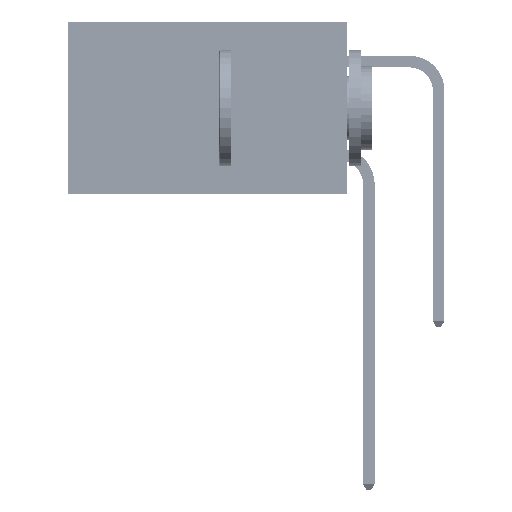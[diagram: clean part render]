
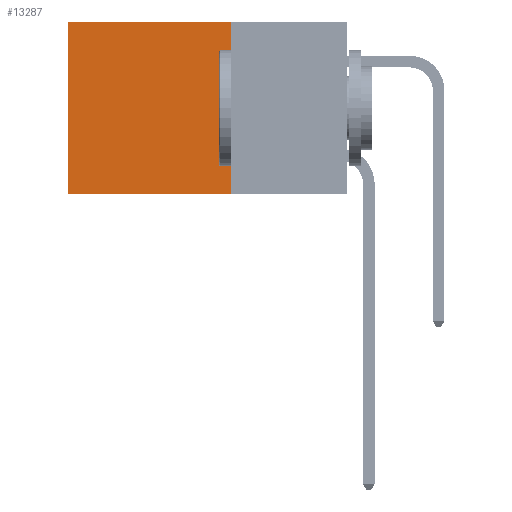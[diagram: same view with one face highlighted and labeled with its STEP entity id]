
A CAD part, left-side view. The second image highlights one B-rep face of the part: STEP entity #13287.
In plain terms, the highlighted planar face has unit normal (-1, 0, 0).
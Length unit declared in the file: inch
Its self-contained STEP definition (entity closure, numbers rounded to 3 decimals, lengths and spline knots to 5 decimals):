
#1225 = CARTESIAN_POINT ( 'NONE',  ( 0.2875, 0.25, 0. ) ) ;
#5176 = VERTEX_POINT ( 'NONE', #8591 ) ;
#8591 = CARTESIAN_POINT ( 'NONE',  ( 0.2875, 0.6, 0. ) ) ;
#10971 = DIRECTION ( 'NONE',  ( 0., 1., 0. ) ) ;
#11644 = CARTESIAN_POINT ( 'NONE',  ( 0.2875, 0.6, 0. ) ) ;
#11770 = DIRECTION ( 'NONE',  ( 0., 1., 0. ) ) ;
#12462 = DIRECTION ( 'NONE',  ( 0., 0., -1. ) ) ;
#12491 = VERTEX_POINT ( 'NONE', #29172 ) ;
#13287 = ADVANCED_FACE ( 'NONE', ( #17863 ), #16304, .F. ) ;
#14260 = CARTESIAN_POINT ( 'NONE',  ( 0.2875, 0.25, -0.37 ) ) ;
#14838 = LINE ( 'NONE', #1225, #18210 ) ;
#16304 = PLANE ( 'NONE',  #39725 ) ;
#16972 = ORIENTED_EDGE ( 'NONE', *, *, #40409, .T. ) ;
#17863 = FACE_OUTER_BOUND ( 'NONE', #26977, .T. ) ;
#18210 = VECTOR ( 'NONE', #12462, 39.37008 ) ;
#18788 = DIRECTION ( 'NONE',  ( 1., 0., 0. ) ) ;
#20261 = ORIENTED_EDGE ( 'NONE', *, *, #29872, .T. ) ;
#22679 = VECTOR ( 'NONE', #29223, 39.37008 ) ;
#23508 = CARTESIAN_POINT ( 'NONE',  ( 0.2875, 0.25, 0. ) ) ;
#23659 = CARTESIAN_POINT ( 'NONE',  ( 0.2875, 0.6, -0.37 ) ) ;
#25288 = CARTESIAN_POINT ( 'NONE',  ( 0.2875, 0.25, -0.37 ) ) ;
#25747 = LINE ( 'NONE', #25288, #45305 ) ;
#26019 = DIRECTION ( 'NONE',  ( 0., 0., -1. ) ) ;
#26977 = EDGE_LOOP ( 'NONE', ( #20261, #38622, #41248, #16972 ) ) ;
#29172 = CARTESIAN_POINT ( 'NONE',  ( 0.2875, 0.25, 0. ) ) ;
#29223 = DIRECTION ( 'NONE',  ( 0., 0., -1. ) ) ;
#29872 = EDGE_CURVE ( 'NONE', #5176, #43498, #43297, .T. ) ;
#32096 = VECTOR ( 'NONE', #11770, 39.37008 ) ;
#32393 = EDGE_CURVE ( 'NONE', #33013, #43498, #25747, .T. ) ;
#33013 = VERTEX_POINT ( 'NONE', #14260 ) ;
#33671 = CARTESIAN_POINT ( 'NONE',  ( 0.2875, 0.25, 0. ) ) ;
#38622 = ORIENTED_EDGE ( 'NONE', *, *, #32393, .F. ) ;
#39725 = AXIS2_PLACEMENT_3D ( 'NONE', #23508, #18788, #26019 ) ;
#39783 = EDGE_CURVE ( 'NONE', #12491, #33013, #14838, .T. ) ;
#39956 = LINE ( 'NONE', #33671, #32096 ) ;
#40409 = EDGE_CURVE ( 'NONE', #12491, #5176, #39956, .T. ) ;
#41248 = ORIENTED_EDGE ( 'NONE', *, *, #39783, .F. ) ;
#43297 = LINE ( 'NONE', #11644, #22679 ) ;
#43498 = VERTEX_POINT ( 'NONE', #23659 ) ;
#45305 = VECTOR ( 'NONE', #10971, 39.37008 ) ;
